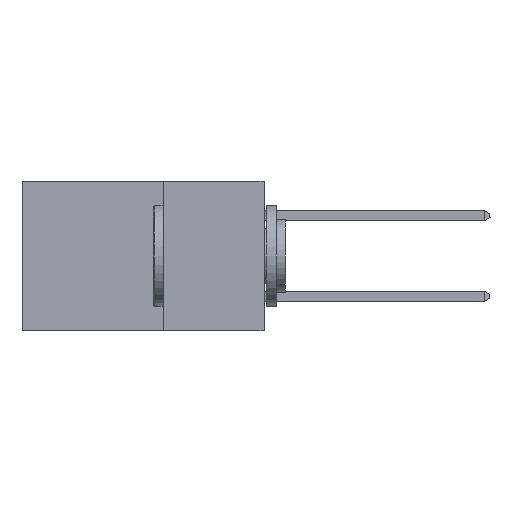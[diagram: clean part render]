
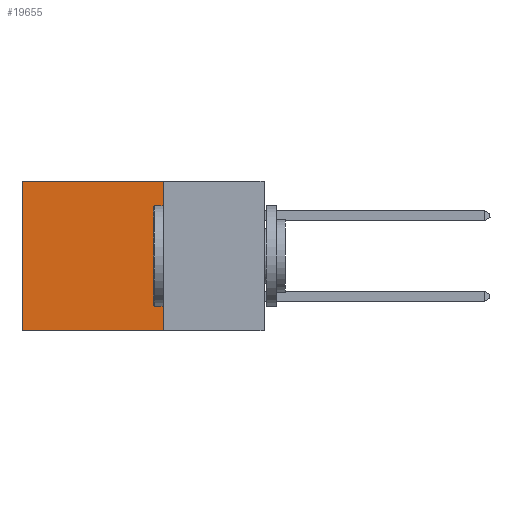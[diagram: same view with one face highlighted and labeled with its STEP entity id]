
A CAD part, left-side view. The second image highlights one B-rep face of the part: STEP entity #19655.
In plain terms, the highlighted planar face has unit normal (-1, 0, 0).
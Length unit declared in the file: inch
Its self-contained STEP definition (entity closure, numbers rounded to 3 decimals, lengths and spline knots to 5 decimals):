
#2115 = EDGE_CURVE ( 'NONE', #7337, #17811, #19217, .T. ) ;
#2189 = ORIENTED_EDGE ( 'NONE', *, *, #8383, .T. ) ;
#2804 = EDGE_CURVE ( 'NONE', #15166, #17811, #16016, .T. ) ;
#3122 = AXIS2_PLACEMENT_3D ( 'NONE', #13785, #4390, #15508 ) ;
#3527 = EDGE_CURVE ( 'NONE', #5054, #15166, #4174, .T. ) ;
#4174 = LINE ( 'NONE', #11062, #18632 ) ;
#4390 = DIRECTION ( 'NONE',  ( 1., 0., 0. ) ) ;
#4690 = VECTOR ( 'NONE', #8446, 39.37008 ) ;
#5054 = VERTEX_POINT ( 'NONE', #16916 ) ;
#5252 = ORIENTED_EDGE ( 'NONE', *, *, #3527, .F. ) ;
#6176 = ORIENTED_EDGE ( 'NONE', *, *, #2115, .T. ) ;
#7337 = VERTEX_POINT ( 'NONE', #9631 ) ;
#8027 = EDGE_LOOP ( 'NONE', ( #6176, #11404, #5252, #2189 ) ) ;
#8383 = EDGE_CURVE ( 'NONE', #5054, #7337, #16530, .T. ) ;
#8446 = DIRECTION ( 'NONE',  ( 0., 1., 0. ) ) ;
#9631 = CARTESIAN_POINT ( 'NONE',  ( 0.298, 0.6, 0. ) ) ;
#10877 = VECTOR ( 'NONE', #19360, 39.37008 ) ;
#10986 = CARTESIAN_POINT ( 'NONE',  ( 0.298, 0.25, 0. ) ) ;
#11062 = CARTESIAN_POINT ( 'NONE',  ( 0.298, 0.25, 0. ) ) ;
#11404 = ORIENTED_EDGE ( 'NONE', *, *, #2804, .F. ) ;
#11625 = CARTESIAN_POINT ( 'NONE',  ( 0.298, 0.25, -0.37 ) ) ;
#12909 = FACE_OUTER_BOUND ( 'NONE', #8027, .T. ) ;
#13785 = CARTESIAN_POINT ( 'NONE',  ( 0.298, 0.25, 0. ) ) ;
#14310 = VECTOR ( 'NONE', #20322, 39.37008 ) ;
#14398 = CARTESIAN_POINT ( 'NONE',  ( 0.298, 0.6, -0.37 ) ) ;
#15166 = VERTEX_POINT ( 'NONE', #15880 ) ;
#15508 = DIRECTION ( 'NONE',  ( 0., 0., -1. ) ) ;
#15739 = DIRECTION ( 'NONE',  ( 0., 0., -1. ) ) ;
#15880 = CARTESIAN_POINT ( 'NONE',  ( 0.298, 0.25, -0.37 ) ) ;
#16016 = LINE ( 'NONE', #11625, #4690 ) ;
#16530 = LINE ( 'NONE', #10986, #14310 ) ;
#16916 = CARTESIAN_POINT ( 'NONE',  ( 0.298, 0.25, 0. ) ) ;
#17811 = VERTEX_POINT ( 'NONE', #14398 ) ;
#17921 = CARTESIAN_POINT ( 'NONE',  ( 0.298, 0.6, 0. ) ) ;
#18632 = VECTOR ( 'NONE', #15739, 39.37008 ) ;
#19217 = LINE ( 'NONE', #17921, #10877 ) ;
#19360 = DIRECTION ( 'NONE',  ( 0., 0., -1. ) ) ;
#19655 = ADVANCED_FACE ( 'NONE', ( #12909 ), #20233, .F. ) ;
#20233 = PLANE ( 'NONE',  #3122 ) ;
#20322 = DIRECTION ( 'NONE',  ( 0., 1., 0. ) ) ;
